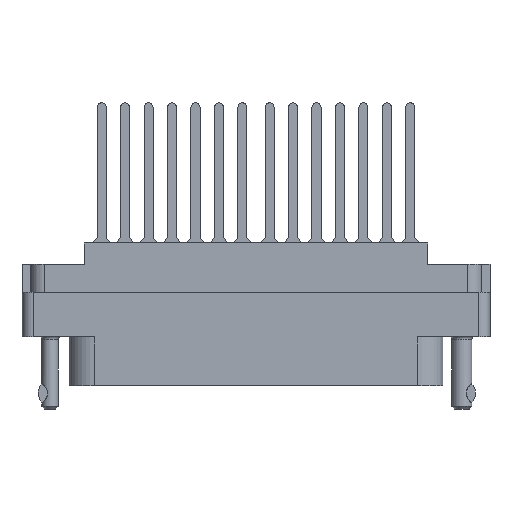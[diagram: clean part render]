
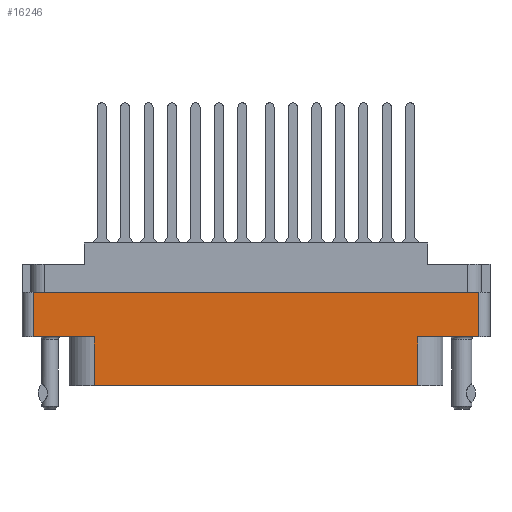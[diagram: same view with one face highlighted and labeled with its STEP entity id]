
A CAD part, front view. The second image highlights one B-rep face of the part: STEP entity #16246.
In plain terms, the highlighted planar face has unit normal (0, -1, 0).
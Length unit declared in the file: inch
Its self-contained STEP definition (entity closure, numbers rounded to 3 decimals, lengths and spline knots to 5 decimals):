
#317 = EDGE_CURVE ( 'NONE', #5036, #17654, #15615, .T. ) ;
#2106 = DIRECTION ( 'NONE',  ( 1., 0., 0. ) ) ;
#3357 = ORIENTED_EDGE ( 'NONE', *, *, #17091, .F. ) ;
#3366 = CARTESIAN_POINT ( 'NONE',  ( 1.2335, -0.438, -0.52 ) ) ;
#3607 = DIRECTION ( 'NONE',  ( 0., -1., 0. ) ) ;
#5035 = DIRECTION ( 'NONE',  ( 0., 0., 1. ) ) ;
#5036 = VERTEX_POINT ( 'NONE', #3366 ) ;
#6745 = VECTOR ( 'NONE', #19839, 39.37008 ) ;
#9905 = DIRECTION ( 'NONE',  ( -1., 0., 0. ) ) ;
#10315 = DIRECTION ( 'NONE',  ( -1., 0., 0. ) ) ;
#11907 = CARTESIAN_POINT ( 'NONE',  ( 1.2335, -0.438, -0.274 ) ) ;
#11984 = DIRECTION ( 'NONE',  ( 0., 0., -1. ) ) ;
#12632 = EDGE_CURVE ( 'NONE', #55780, #35124, #29609, .T. ) ;
#13012 = EDGE_CURVE ( 'NONE', #55780, #56620, #29550, .T. ) ;
#15615 = LINE ( 'NONE', #27855, #26164 ) ;
#16246 = ADVANCED_FACE ( 'NONE', ( #39784 ), #35744, .T. ) ;
#16465 = VERTEX_POINT ( 'NONE', #52688 ) ;
#16983 = LINE ( 'NONE', #39065, #25475 ) ;
#17091 = EDGE_CURVE ( 'NONE', #57788, #38847, #22715, .T. ) ;
#17654 = VERTEX_POINT ( 'NONE', #18753 ) ;
#17973 = CARTESIAN_POINT ( 'NONE',  ( -1.2335, -0.438, -0.274 ) ) ;
#18167 = ORIENTED_EDGE ( 'NONE', *, *, #317, .F. ) ;
#18753 = CARTESIAN_POINT ( 'NONE',  ( 0.895, -0.438, -0.52 ) ) ;
#18874 = LINE ( 'NONE', #32197, #31616 ) ;
#19110 = AXIS2_PLACEMENT_3D ( 'NONE', #31594, #3607, #31395 ) ;
#19839 = DIRECTION ( 'NONE',  ( 0., 0., 1. ) ) ;
#20035 = CARTESIAN_POINT ( 'NONE',  ( 1.2335, -0.438, -0.789 ) ) ;
#20952 = VECTOR ( 'NONE', #2106, 39.37008 ) ;
#21031 = DIRECTION ( 'NONE',  ( 1., 0., 0. ) ) ;
#21686 = LINE ( 'NONE', #28309, #20952 ) ;
#22715 = LINE ( 'NONE', #39257, #53121 ) ;
#23392 = ORIENTED_EDGE ( 'NONE', *, *, #13012, .F. ) ;
#24335 = ORIENTED_EDGE ( 'NONE', *, *, #12632, .T. ) ;
#25475 = VECTOR ( 'NONE', #11984, 39.37008 ) ;
#25834 = LINE ( 'NONE', #20035, #6745 ) ;
#26067 = ORIENTED_EDGE ( 'NONE', *, *, #29225, .T. ) ;
#26164 = VECTOR ( 'NONE', #9905, 39.37008 ) ;
#27236 = ORIENTED_EDGE ( 'NONE', *, *, #31330, .T. ) ;
#27855 = CARTESIAN_POINT ( 'NONE',  ( 0., -0.438, -0.52 ) ) ;
#28309 = CARTESIAN_POINT ( 'NONE',  ( -1.2955, -0.438, -0.789 ) ) ;
#28451 = CARTESIAN_POINT ( 'NONE',  ( 0., -0.438, -0.52 ) ) ;
#29225 = EDGE_CURVE ( 'NONE', #57788, #56620, #16983, .T. ) ;
#29453 = EDGE_LOOP ( 'NONE', ( #3357, #26067, #23392, #24335, #44515, #27236, #18167, #33756 ) ) ;
#29550 = LINE ( 'NONE', #28451, #57857 ) ;
#29609 = LINE ( 'NONE', #55684, #30311 ) ;
#30311 = VECTOR ( 'NONE', #33486, 39.37008 ) ;
#31330 = EDGE_CURVE ( 'NONE', #16465, #17654, #18874, .T. ) ;
#31395 = DIRECTION ( 'NONE',  ( 0., 0., -1. ) ) ;
#31594 = CARTESIAN_POINT ( 'NONE',  ( -1.2955, -0.438, -0.789 ) ) ;
#31616 = VECTOR ( 'NONE', #5035, 39.37008 ) ;
#32197 = CARTESIAN_POINT ( 'NONE',  ( 0.895, -0.438, -0.52 ) ) ;
#33486 = DIRECTION ( 'NONE',  ( 0., 0., -1. ) ) ;
#33756 = ORIENTED_EDGE ( 'NONE', *, *, #50272, .T. ) ;
#35124 = VERTEX_POINT ( 'NONE', #38584 ) ;
#35744 = PLANE ( 'NONE',  #19110 ) ;
#38584 = CARTESIAN_POINT ( 'NONE',  ( -0.895, -0.438, -0.789 ) ) ;
#38847 = VERTEX_POINT ( 'NONE', #11907 ) ;
#39065 = CARTESIAN_POINT ( 'NONE',  ( -1.2335, -0.438, -0.789 ) ) ;
#39257 = CARTESIAN_POINT ( 'NONE',  ( 0., -0.438, -0.274 ) ) ;
#39784 = FACE_OUTER_BOUND ( 'NONE', #29453, .T. ) ;
#44515 = ORIENTED_EDGE ( 'NONE', *, *, #56913, .T. ) ;
#50272 = EDGE_CURVE ( 'NONE', #5036, #38847, #25834, .T. ) ;
#52688 = CARTESIAN_POINT ( 'NONE',  ( 0.895, -0.438, -0.789 ) ) ;
#53121 = VECTOR ( 'NONE', #21031, 39.37008 ) ;
#55684 = CARTESIAN_POINT ( 'NONE',  ( -0.895, -0.438, -0.789 ) ) ;
#55780 = VERTEX_POINT ( 'NONE', #55886 ) ;
#55886 = CARTESIAN_POINT ( 'NONE',  ( -0.895, -0.438, -0.52 ) ) ;
#56620 = VERTEX_POINT ( 'NONE', #57201 ) ;
#56913 = EDGE_CURVE ( 'NONE', #35124, #16465, #21686, .T. ) ;
#57201 = CARTESIAN_POINT ( 'NONE',  ( -1.2335, -0.438, -0.52 ) ) ;
#57788 = VERTEX_POINT ( 'NONE', #17973 ) ;
#57857 = VECTOR ( 'NONE', #10315, 39.37008 ) ;
